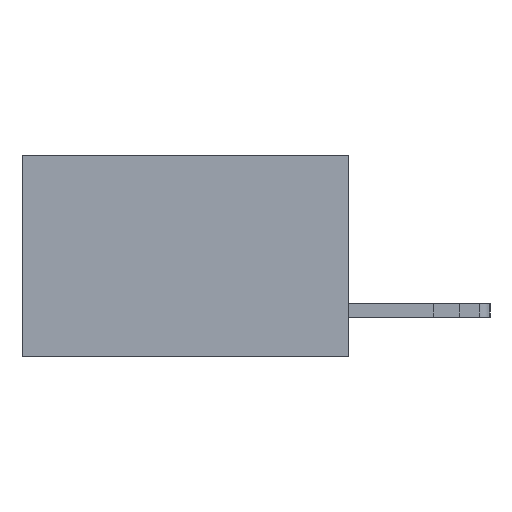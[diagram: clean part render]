
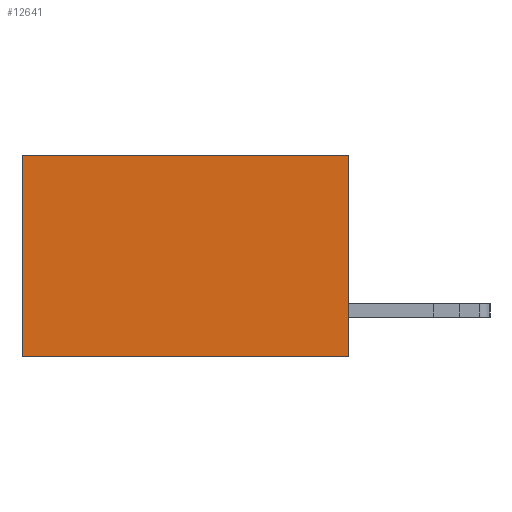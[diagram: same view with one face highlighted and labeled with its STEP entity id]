
A CAD part, left-side view. The second image highlights one B-rep face of the part: STEP entity #12641.
In plain terms, the highlighted planar face has unit normal (-1, 0, 0).
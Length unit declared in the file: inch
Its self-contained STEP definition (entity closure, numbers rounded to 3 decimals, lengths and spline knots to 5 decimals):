
#224 = VERTEX_POINT ( 'NONE', #12029 ) ;
#2091 = CARTESIAN_POINT ( 'NONE',  ( 0.298, 0., 0. ) ) ;
#2326 = LINE ( 'NONE', #2091, #8299 ) ;
#2900 = CARTESIAN_POINT ( 'NONE',  ( 0.298, 0., 0. ) ) ;
#3040 = EDGE_CURVE ( 'NONE', #9039, #224, #2326, .T. ) ;
#3382 = LINE ( 'NONE', #8826, #13741 ) ;
#3420 = DIRECTION ( 'NONE',  ( 0., 0., -1. ) ) ;
#3599 = LINE ( 'NONE', #5190, #9962 ) ;
#3846 = EDGE_CURVE ( 'NONE', #9039, #11122, #3599, .T. ) ;
#4161 = CARTESIAN_POINT ( 'NONE',  ( 0.298, 0., -0.37 ) ) ;
#4301 = DIRECTION ( 'NONE',  ( 1., 0., 0. ) ) ;
#5190 = CARTESIAN_POINT ( 'NONE',  ( 0.298, 0., 0. ) ) ;
#6046 = VECTOR ( 'NONE', #12212, 39.37008 ) ;
#7362 = ORIENTED_EDGE ( 'NONE', *, *, #3846, .F. ) ;
#8165 = DIRECTION ( 'NONE',  ( 0., 0., -1. ) ) ;
#8299 = VECTOR ( 'NONE', #14959, 39.37008 ) ;
#8431 = ORIENTED_EDGE ( 'NONE', *, *, #9219, .F. ) ;
#8826 = CARTESIAN_POINT ( 'NONE',  ( 0.298, 0.6, 0. ) ) ;
#9039 = VERTEX_POINT ( 'NONE', #9195 ) ;
#9195 = CARTESIAN_POINT ( 'NONE',  ( 0.298, 0., 0. ) ) ;
#9219 = EDGE_CURVE ( 'NONE', #11122, #12777, #12750, .T. ) ;
#9962 = VECTOR ( 'NONE', #8165, 39.37008 ) ;
#11122 = VERTEX_POINT ( 'NONE', #12397 ) ;
#11852 = AXIS2_PLACEMENT_3D ( 'NONE', #2900, #4301, #13717 ) ;
#12029 = CARTESIAN_POINT ( 'NONE',  ( 0.298, 0.6, 0. ) ) ;
#12212 = DIRECTION ( 'NONE',  ( 0., 1., 0. ) ) ;
#12351 = PLANE ( 'NONE',  #11852 ) ;
#12397 = CARTESIAN_POINT ( 'NONE',  ( 0.298, 0., -0.37 ) ) ;
#12641 = ADVANCED_FACE ( 'NONE', ( #17044 ), #12351, .F. ) ;
#12750 = LINE ( 'NONE', #4161, #6046 ) ;
#12777 = VERTEX_POINT ( 'NONE', #13939 ) ;
#13717 = DIRECTION ( 'NONE',  ( 0., 0., -1. ) ) ;
#13741 = VECTOR ( 'NONE', #3420, 39.37008 ) ;
#13939 = CARTESIAN_POINT ( 'NONE',  ( 0.298, 0.6, -0.37 ) ) ;
#14089 = EDGE_CURVE ( 'NONE', #224, #12777, #3382, .T. ) ;
#14317 = ORIENTED_EDGE ( 'NONE', *, *, #3040, .T. ) ;
#14665 = ORIENTED_EDGE ( 'NONE', *, *, #14089, .T. ) ;
#14959 = DIRECTION ( 'NONE',  ( 0., 1., 0. ) ) ;
#16493 = EDGE_LOOP ( 'NONE', ( #14665, #8431, #7362, #14317 ) ) ;
#17044 = FACE_OUTER_BOUND ( 'NONE', #16493, .T. ) ;
